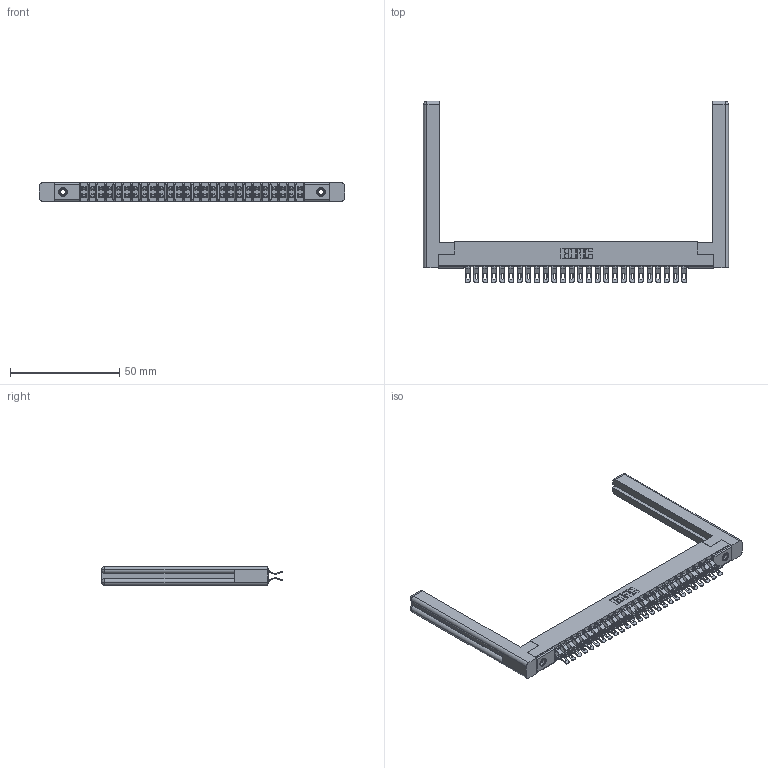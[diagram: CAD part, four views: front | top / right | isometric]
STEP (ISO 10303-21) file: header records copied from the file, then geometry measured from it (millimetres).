
FILE_DESCRIPTION (( 'STEP AP203' ), '1' );
FILE_NAME ('307-052-555-258.STEP', '2019-09-06T12:20:45', ( '' ), ( '' ), 'SwSTEP 2.0', 'SolidWorks 2016', '' );
FILE_SCHEMA (( 'CONFIG_CONTROL_DESIGN' ));
Length unit declared in the file: inch
Products named in the file (5): 307-220-058; 345-250-001_345-250-001-102; 307-052-555-258; 307-290-001_555; 307 Part_.156 Dia Mounting Holes
Assembly tree (57 placements, depth 2):
  307-052-555-258
    307 Part_.156 Dia Mounting Holes
    307-290-001_555  x52
    307-220-058  x2
    345-250-001_345-250-001-102  x2
Bounding box: 139.65 x 83.06 x 8.71 mm (x, y, z)
Volume: 16975.7 mm3; surface area: 22560.5 mm2
Topology: 57 solids, 57 shells, 3459 faces, 10089 edges, 6570 vertices
Faces by surface type: plane 1922, cylinder 1459, sphere 54, torus 12, cone 12
Entity records: 28264 total; most frequent: CARTESIAN_POINT 4653, ORIENTED_EDGE 4554, DIRECTION 4529, EDGE_CURVE 2277, LINE 1725, VECTOR 1725, VERTEX_POINT 1472, AXIS2_PLACEMENT_3D 1402
